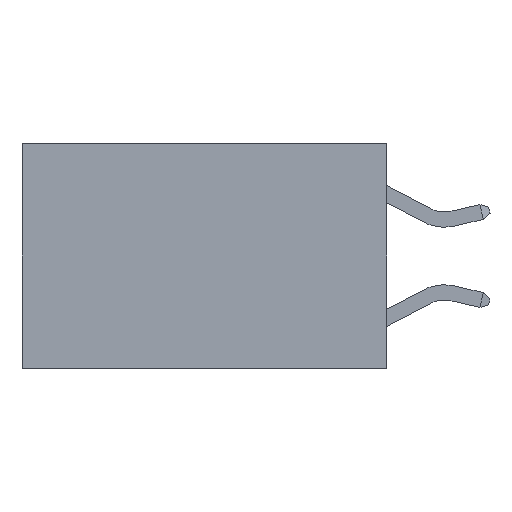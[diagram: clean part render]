
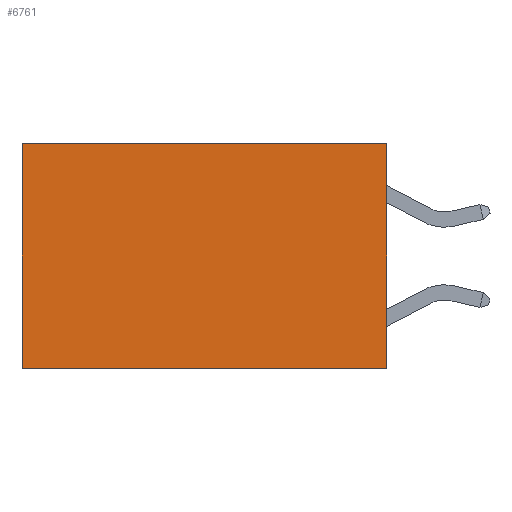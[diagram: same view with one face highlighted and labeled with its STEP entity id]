
A CAD part, left-side view. The second image highlights one B-rep face of the part: STEP entity #6761.
In plain terms, the highlighted planar face has unit normal (-1, 0, 0).
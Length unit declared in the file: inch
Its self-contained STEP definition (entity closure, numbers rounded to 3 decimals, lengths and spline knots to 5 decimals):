
#1360 = DIRECTION ( 'NONE',  ( 0., 1., 0. ) ) ;
#2126 = EDGE_CURVE ( 'NONE', #17511, #25357, #26707, .T. ) ;
#3587 = ORIENTED_EDGE ( 'NONE', *, *, #19775, .T. ) ;
#4074 = PLANE ( 'NONE',  #18207 ) ;
#4442 = ORIENTED_EDGE ( 'NONE', *, *, #6459, .T. ) ;
#4466 = CARTESIAN_POINT ( 'NONE',  ( 0.2625, 0., 0. ) ) ;
#5824 = VECTOR ( 'NONE', #24509, 39.37008 ) ;
#6028 = CARTESIAN_POINT ( 'NONE',  ( 0.2625, 0.6, 0. ) ) ;
#6168 = DIRECTION ( 'NONE',  ( 0., 0., -1. ) ) ;
#6236 = DIRECTION ( 'NONE',  ( 1., 0., 0. ) ) ;
#6459 = EDGE_CURVE ( 'NONE', #20616, #25357, #24956, .T. ) ;
#6761 = ADVANCED_FACE ( 'NONE', ( #18894 ), #4074, .F. ) ;
#9775 = VECTOR ( 'NONE', #1360, 39.37008 ) ;
#11099 = CARTESIAN_POINT ( 'NONE',  ( 0.2625, 0., -0.37 ) ) ;
#11448 = LINE ( 'NONE', #24081, #9775 ) ;
#13964 = DIRECTION ( 'NONE',  ( 0., 1., 0. ) ) ;
#15001 = ORIENTED_EDGE ( 'NONE', *, *, #19493, .F. ) ;
#15834 = CARTESIAN_POINT ( 'NONE',  ( 0.2625, 0.6, 0. ) ) ;
#16341 = LINE ( 'NONE', #22477, #5824 ) ;
#17511 = VERTEX_POINT ( 'NONE', #11099 ) ;
#18207 = AXIS2_PLACEMENT_3D ( 'NONE', #4466, #6236, #23120 ) ;
#18894 = FACE_OUTER_BOUND ( 'NONE', #22674, .T. ) ;
#19493 = EDGE_CURVE ( 'NONE', #20032, #17511, #16341, .T. ) ;
#19775 = EDGE_CURVE ( 'NONE', #20032, #20616, #11448, .T. ) ;
#20032 = VERTEX_POINT ( 'NONE', #22699 ) ;
#20616 = VERTEX_POINT ( 'NONE', #15834 ) ;
#21580 = CARTESIAN_POINT ( 'NONE',  ( 0.2625, 0.6, -0.37 ) ) ;
#22122 = CARTESIAN_POINT ( 'NONE',  ( 0.2625, 0., -0.37 ) ) ;
#22477 = CARTESIAN_POINT ( 'NONE',  ( 0.2625, 0., 0. ) ) ;
#22674 = EDGE_LOOP ( 'NONE', ( #4442, #22767, #15001, #3587 ) ) ;
#22699 = CARTESIAN_POINT ( 'NONE',  ( 0.2625, 0., 0. ) ) ;
#22767 = ORIENTED_EDGE ( 'NONE', *, *, #2126, .F. ) ;
#23120 = DIRECTION ( 'NONE',  ( 0., 0., -1. ) ) ;
#23523 = VECTOR ( 'NONE', #6168, 39.37008 ) ;
#24081 = CARTESIAN_POINT ( 'NONE',  ( 0.2625, 0., 0. ) ) ;
#24509 = DIRECTION ( 'NONE',  ( 0., 0., -1. ) ) ;
#24956 = LINE ( 'NONE', #6028, #23523 ) ;
#25357 = VERTEX_POINT ( 'NONE', #21580 ) ;
#26286 = VECTOR ( 'NONE', #13964, 39.37008 ) ;
#26707 = LINE ( 'NONE', #22122, #26286 ) ;
